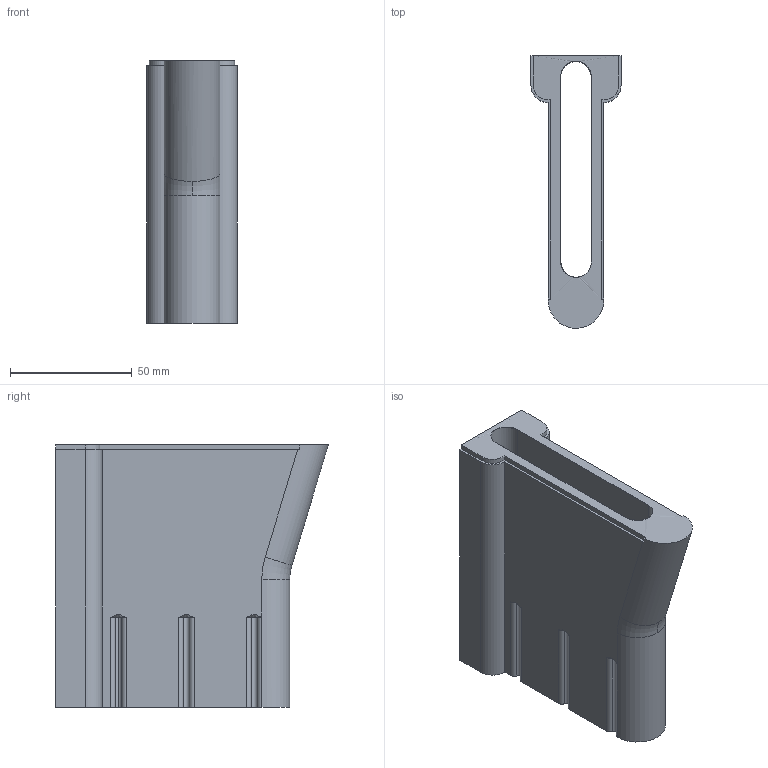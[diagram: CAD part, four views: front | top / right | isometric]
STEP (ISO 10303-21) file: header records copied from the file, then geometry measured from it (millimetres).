
FILE_DESCRIPTION (( 'STEP AP214' ), '1' );
FILE_NAME ('Charon_V3_Rifle_2_1.step', '2019-12-18T03:07:35', ( '' ), ( '' ), 'SwSTEP 2.0', 'SolidWorks 2019', '' );
FILE_SCHEMA (( 'AUTOMOTIVE_DESIGN' ));
Length unit declared in the file: millimetre
Products named in the file (1): Charon_V3_Rifle_2_1
Bounding box: 37.13 x 112.17 x 108 mm (x, y, z)
Volume: 149056.3 mm3; surface area: 52566.6 mm2
Topology: 1 solids, 1 shells, 129 faces, 430 edges, 269 vertices
Faces by surface type: sphere 50, cylinder 32, plane 23, cone 22, torus 2
Entity records: 3934 total; most frequent: DIRECTION 742, CARTESIAN_POINT 715, ORIENTED_EDGE 628, AXIS2_PLACEMENT_3D 318, EDGE_CURVE 314, VERTEX_POINT 211, CIRCLE 188, EDGE_LOOP 155
